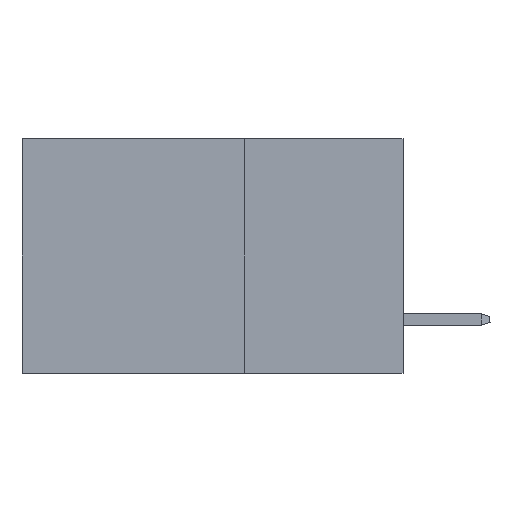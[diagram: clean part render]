
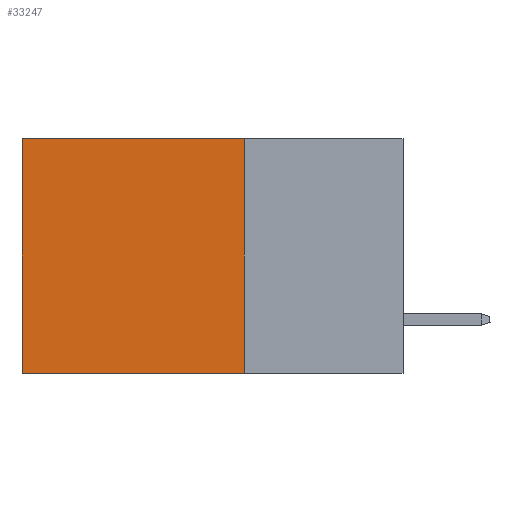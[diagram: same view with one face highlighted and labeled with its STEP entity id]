
A CAD part, left-side view. The second image highlights one B-rep face of the part: STEP entity #33247.
In plain terms, the highlighted planar face has unit normal (-1, 0, 0).
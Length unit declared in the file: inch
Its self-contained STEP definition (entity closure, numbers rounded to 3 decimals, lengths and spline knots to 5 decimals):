
#768 = DIRECTION ( 'NONE',  ( 1., 0., 0. ) ) ;
#1588 = VECTOR ( 'NONE', #33246, 39.37008 ) ;
#3502 = VECTOR ( 'NONE', #12712, 39.37008 ) ;
#5766 = ORIENTED_EDGE ( 'NONE', *, *, #16689, .F. ) ;
#6510 = LINE ( 'NONE', #9793, #3502 ) ;
#6887 = VERTEX_POINT ( 'NONE', #12009 ) ;
#8581 = CARTESIAN_POINT ( 'NONE',  ( 0.2875, 0.6, -0.37 ) ) ;
#9793 = CARTESIAN_POINT ( 'NONE',  ( 0.2875, 0.25, 0. ) ) ;
#12009 = CARTESIAN_POINT ( 'NONE',  ( 0.2875, 0.25, -0.37 ) ) ;
#12712 = DIRECTION ( 'NONE',  ( 0., 1., 0. ) ) ;
#13671 = ORIENTED_EDGE ( 'NONE', *, *, #14461, .T. ) ;
#14060 = LINE ( 'NONE', #22093, #24611 ) ;
#14461 = EDGE_CURVE ( 'NONE', #19241, #17859, #6510, .T. ) ;
#14625 = CARTESIAN_POINT ( 'NONE',  ( 0.2875, 0.25, 0. ) ) ;
#16689 = EDGE_CURVE ( 'NONE', #19241, #6887, #14060, .T. ) ;
#17859 = VERTEX_POINT ( 'NONE', #30118 ) ;
#18772 = LINE ( 'NONE', #26956, #26511 ) ;
#19241 = VERTEX_POINT ( 'NONE', #33083 ) ;
#19745 = DIRECTION ( 'NONE',  ( 0., 0., -1. ) ) ;
#20658 = EDGE_CURVE ( 'NONE', #6887, #26987, #18772, .T. ) ;
#22093 = CARTESIAN_POINT ( 'NONE',  ( 0.2875, 0.25, 0. ) ) ;
#22142 = CARTESIAN_POINT ( 'NONE',  ( 0.2875, 0.6, 0. ) ) ;
#22714 = ORIENTED_EDGE ( 'NONE', *, *, #23035, .T. ) ;
#23015 = FACE_OUTER_BOUND ( 'NONE', #34388, .T. ) ;
#23035 = EDGE_CURVE ( 'NONE', #17859, #26987, #24877, .T. ) ;
#24611 = VECTOR ( 'NONE', #33195, 39.37008 ) ;
#24877 = LINE ( 'NONE', #22142, #1588 ) ;
#26511 = VECTOR ( 'NONE', #35698, 39.37008 ) ;
#26956 = CARTESIAN_POINT ( 'NONE',  ( 0.2875, 0.25, -0.37 ) ) ;
#26987 = VERTEX_POINT ( 'NONE', #8581 ) ;
#27305 = ORIENTED_EDGE ( 'NONE', *, *, #20658, .F. ) ;
#30118 = CARTESIAN_POINT ( 'NONE',  ( 0.2875, 0.6, 0. ) ) ;
#33083 = CARTESIAN_POINT ( 'NONE',  ( 0.2875, 0.25, 0. ) ) ;
#33195 = DIRECTION ( 'NONE',  ( 0., 0., -1. ) ) ;
#33246 = DIRECTION ( 'NONE',  ( 0., 0., -1. ) ) ;
#33247 = ADVANCED_FACE ( 'NONE', ( #23015 ), #34120, .F. ) ;
#34120 = PLANE ( 'NONE',  #35120 ) ;
#34388 = EDGE_LOOP ( 'NONE', ( #22714, #27305, #5766, #13671 ) ) ;
#35120 = AXIS2_PLACEMENT_3D ( 'NONE', #14625, #768, #19745 ) ;
#35698 = DIRECTION ( 'NONE',  ( 0., 1., 0. ) ) ;
